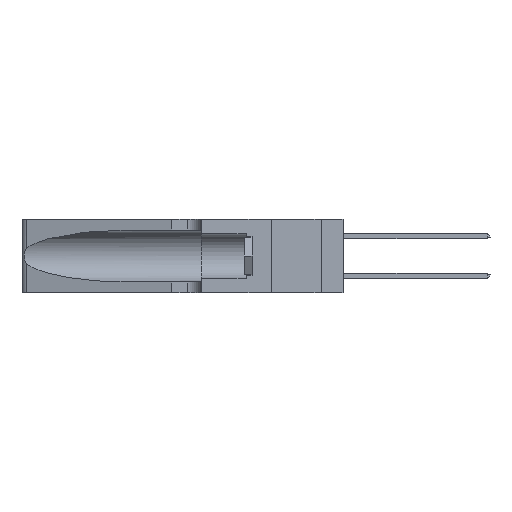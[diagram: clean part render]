
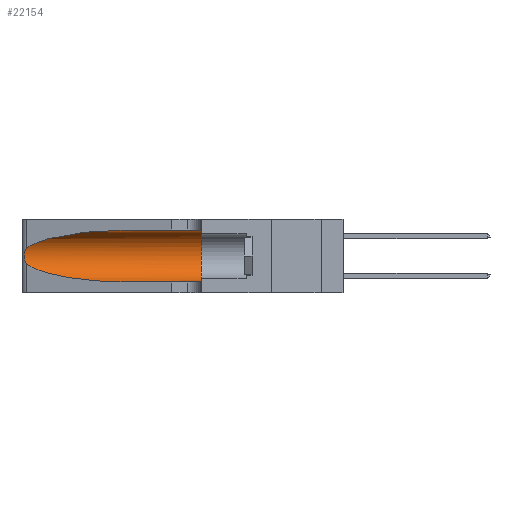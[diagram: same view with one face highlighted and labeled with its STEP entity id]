
A CAD part, left-side view. The second image highlights one B-rep face of the part: STEP entity #22154.
In plain terms, the highlighted cylindrical face has radius 3.308 mm (diameter 6.617 mm), a partial arc.
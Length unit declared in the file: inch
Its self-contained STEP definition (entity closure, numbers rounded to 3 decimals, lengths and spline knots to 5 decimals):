
#251 = CARTESIAN_POINT ( 'NONE',  ( 0.25787, 1.23484, 0.2124 ) ) ;
#449 = CARTESIAN_POINT ( 'NONE',  ( 0.1305, 0.35, 0.185 ) ) ;
#828 = DIRECTION ( 'NONE',  ( 0., -1., 0. ) ) ;
#871 = FACE_OUTER_BOUND ( 'NONE', #7618, .T. ) ;
#877 = DIRECTION ( 'NONE',  ( 0., -1., 0. ) ) ;
#981 = CARTESIAN_POINT ( 'NONE',  ( 0.25487, 1.22718, 0.14631 ) ) ;
#1498 = ORIENTED_EDGE ( 'NONE', *, *, #20898, .F. ) ;
#2138 = CARTESIAN_POINT ( 'NONE',  ( 0.26018, 1.23835, 0.19895 ) ) ;
#2320 = DIRECTION ( 'NONE',  ( 0., 0., 1. ) ) ;
#2988 =( BOUNDED_CURVE ( )  B_SPLINE_CURVE ( 3, ( #11115, #19617, #16303, #5794 ),
 .UNSPECIFIED., .F., .T. ) 
 B_SPLINE_CURVE_WITH_KNOTS ( ( 4, 4 ),
 ( 3.44316, 4.71239 ),
 .UNSPECIFIED. ) 
 CURVE ( )  GEOMETRIC_REPRESENTATION_ITEM ( )  RATIONAL_B_SPLINE_CURVE ( ( 1., 0.87, 0.87, 1. ) ) 
 REPRESENTATION_ITEM ( '' )  );
#3228 = ORIENTED_EDGE ( 'NONE', *, *, #7362, .F. ) ;
#3308 = VERTEX_POINT ( 'NONE', #16849 ) ;
#3512 = VERTEX_POINT ( 'NONE', #22357 ) ;
#3886 = CARTESIAN_POINT ( 'NONE',  ( 0.25487, 1.22718, 0.22369 ) ) ;
#3960 = CARTESIAN_POINT ( 'NONE',  ( 0.26075, 1.23896, 0.178 ) ) ;
#3999 = B_SPLINE_CURVE_WITH_KNOTS ( 'NONE', 3,
 ( #3886, #19622, #11119, #251, #12836, #2138, #14559, #3960, #16305, #5797, #18006, #7609, #19699, #9403 ),
 .UNSPECIFIED., .F., .F.,
 ( 4, 2, 2, 2, 2, 2, 4 ),
 ( 0., 0.00027, 0.00053, 0.00107, 0.0016, 0.00187, 0.00214 ),
 .UNSPECIFIED. ) ;
#4437 =( BOUNDED_CURVE ( )  B_SPLINE_CURVE ( 3, ( #6957, #5134, #17383, #19070 ),
 .UNSPECIFIED., .F., .F. ) 
 B_SPLINE_CURVE_WITH_KNOTS ( ( 4, 4 ),
 ( 1.5708, 2.84003 ),
 .UNSPECIFIED. ) 
 CURVE ( )  GEOMETRIC_REPRESENTATION_ITEM ( )  RATIONAL_B_SPLINE_CURVE ( ( 1., 0.87, 0.87, 1. ) ) 
 REPRESENTATION_ITEM ( '' )  );
#4771 = EDGE_CURVE ( 'NONE', #20207, #8926, #4437, .T. ) ;
#5134 = CARTESIAN_POINT ( 'NONE',  ( 0.18966, 0.96281, 0.31525 ) ) ;
#5480 = CIRCLE ( 'NONE', #8275, 0.13025 ) ;
#5596 = DIRECTION ( 'NONE',  ( 0., -1., 0. ) ) ;
#5794 = CARTESIAN_POINT ( 'NONE',  ( 0.1305, 0.72297, 0.05475 ) ) ;
#5797 = CARTESIAN_POINT ( 'NONE',  ( 0.25856, 1.23593, 0.16098 ) ) ;
#5893 = CARTESIAN_POINT ( 'NONE',  ( 0.25487, 1.22718, 0.22369 ) ) ;
#6957 = CARTESIAN_POINT ( 'NONE',  ( 0.1305, 0.72297, 0.31525 ) ) ;
#7204 = EDGE_CURVE ( 'NONE', #8926, #16927, #3999, .T. ) ;
#7362 = EDGE_CURVE ( 'NONE', #20207, #3512, #20781, .T. ) ;
#7609 = CARTESIAN_POINT ( 'NONE',  ( 0.25639, 1.23186, 0.15144 ) ) ;
#7618 = EDGE_LOOP ( 'NONE', ( #14766, #10896, #20111, #21468, #1498, #3228 ) ) ;
#8275 = AXIS2_PLACEMENT_3D ( 'NONE', #449, #13018, #2320 ) ;
#8926 = VERTEX_POINT ( 'NONE', #5893 ) ;
#9027 = CARTESIAN_POINT ( 'NONE',  ( 0.1305, 0.72297, 0.31525 ) ) ;
#9202 = CARTESIAN_POINT ( 'NONE',  ( 0.1305, 1.61858, 0.185 ) ) ;
#9403 = CARTESIAN_POINT ( 'NONE',  ( 0.25487, 1.22718, 0.14631 ) ) ;
#9778 = EDGE_CURVE ( 'NONE', #10658, #3308, #17272, .T. ) ;
#10658 = VERTEX_POINT ( 'NONE', #10739 ) ;
#10739 = CARTESIAN_POINT ( 'NONE',  ( 0.1305, 0.72297, 0.05475 ) ) ;
#10896 = ORIENTED_EDGE ( 'NONE', *, *, #7204, .T. ) ;
#10998 = DIRECTION ( 'NONE',  ( 0., 0., -1. ) ) ;
#11115 = CARTESIAN_POINT ( 'NONE',  ( 0.25487, 1.22718, 0.14631 ) ) ;
#11119 = CARTESIAN_POINT ( 'NONE',  ( 0.25639, 1.23184, 0.21858 ) ) ;
#11640 = CARTESIAN_POINT ( 'NONE',  ( 0.1305, 1.61858, 0.31525 ) ) ;
#12272 = VECTOR ( 'NONE', #828, 39.37008 ) ;
#12698 = AXIS2_PLACEMENT_3D ( 'NONE', #9202, #5596, #10998 ) ;
#12836 = CARTESIAN_POINT ( 'NONE',  ( 0.25854, 1.2359, 0.20912 ) ) ;
#13018 = DIRECTION ( 'NONE',  ( 0., 1., 0. ) ) ;
#13127 = EDGE_CURVE ( 'NONE', #16927, #10658, #2988, .T. ) ;
#13413 = CARTESIAN_POINT ( 'NONE',  ( 0.1305, 1.61858, 0.05475 ) ) ;
#14007 = CYLINDRICAL_SURFACE ( 'NONE', #12698, 0.13025 ) ;
#14559 = CARTESIAN_POINT ( 'NONE',  ( 0.26075, 1.23896, 0.19203 ) ) ;
#14766 = ORIENTED_EDGE ( 'NONE', *, *, #4771, .T. ) ;
#16303 = CARTESIAN_POINT ( 'NONE',  ( 0.18966, 0.96281, 0.05475 ) ) ;
#16305 = CARTESIAN_POINT ( 'NONE',  ( 0.26017, 1.23833, 0.17102 ) ) ;
#16849 = CARTESIAN_POINT ( 'NONE',  ( 0.1305, 0.35, 0.05475 ) ) ;
#16927 = VERTEX_POINT ( 'NONE', #981 ) ;
#17272 = LINE ( 'NONE', #13413, #21757 ) ;
#17383 = CARTESIAN_POINT ( 'NONE',  ( 0.2373, 1.15595, 0.28018 ) ) ;
#18006 = CARTESIAN_POINT ( 'NONE',  ( 0.25789, 1.23486, 0.15765 ) ) ;
#19070 = CARTESIAN_POINT ( 'NONE',  ( 0.25487, 1.22718, 0.22369 ) ) ;
#19617 = CARTESIAN_POINT ( 'NONE',  ( 0.2373, 1.15595, 0.08982 ) ) ;
#19622 = CARTESIAN_POINT ( 'NONE',  ( 0.25555, 1.22994, 0.2215 ) ) ;
#19699 = CARTESIAN_POINT ( 'NONE',  ( 0.25555, 1.22993, 0.14849 ) ) ;
#20111 = ORIENTED_EDGE ( 'NONE', *, *, #13127, .T. ) ;
#20207 = VERTEX_POINT ( 'NONE', #9027 ) ;
#20781 = LINE ( 'NONE', #11640, #12272 ) ;
#20898 = EDGE_CURVE ( 'NONE', #3512, #3308, #5480, .T. ) ;
#21468 = ORIENTED_EDGE ( 'NONE', *, *, #9778, .T. ) ;
#21757 = VECTOR ( 'NONE', #877, 39.37008 ) ;
#22154 = ADVANCED_FACE ( 'NONE', ( #871 ), #14007, .F. ) ;
#22357 = CARTESIAN_POINT ( 'NONE',  ( 0.1305, 0.35, 0.31525 ) ) ;
